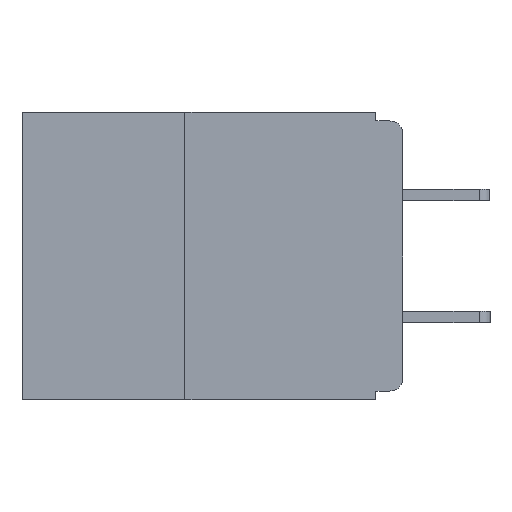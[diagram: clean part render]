
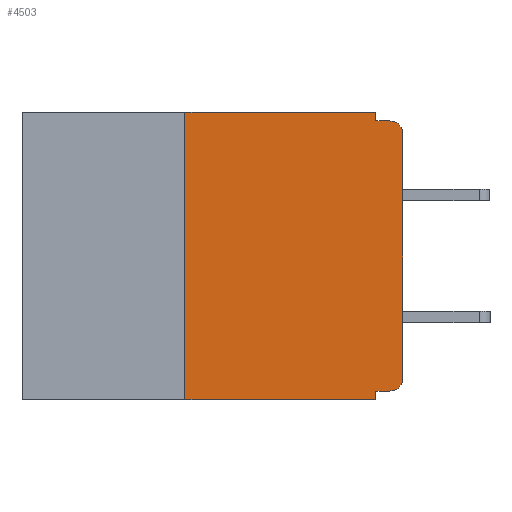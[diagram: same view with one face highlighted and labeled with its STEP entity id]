
A CAD part, left-side view. The second image highlights one B-rep face of the part: STEP entity #4503.
In plain terms, the highlighted planar face has unit normal (-1, 0, 0).
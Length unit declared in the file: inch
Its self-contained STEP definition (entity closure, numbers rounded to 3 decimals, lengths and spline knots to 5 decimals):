
#257 = VERTEX_POINT ( 'NONE', #8727 ) ;
#438 = FACE_OUTER_BOUND ( 'NONE', #10546, .T. ) ;
#1735 = CARTESIAN_POINT ( 'NONE',  ( 0., 0.437, 0. ) ) ;
#1757 = LINE ( 'NONE', #1735, #21112 ) ;
#1858 = LINE ( 'NONE', #15190, #22020 ) ;
#2003 = DIRECTION ( 'NONE',  ( 0., -1., 0. ) ) ;
#3156 = CARTESIAN_POINT ( 'NONE',  ( 0., 0.25, 0. ) ) ;
#3162 = VECTOR ( 'NONE', #19032, 39.37008 ) ;
#3169 = DIRECTION ( 'NONE',  ( 0., 0., -1. ) ) ;
#3252 = ORIENTED_EDGE ( 'NONE', *, *, #29074, .T. ) ;
#3434 = CIRCLE ( 'NONE', #23479, 0.015 ) ;
#4366 = EDGE_CURVE ( 'NONE', #22502, #10629, #18599, .T. ) ;
#4446 = AXIS2_PLACEMENT_3D ( 'NONE', #15179, #31533, #14517 ) ;
#4468 = CARTESIAN_POINT ( 'NONE',  ( 0., 0.031, -0.32 ) ) ;
#4503 = ADVANCED_FACE ( 'NONE', ( #438 ), #16304, .F. ) ;
#4545 = VECTOR ( 'NONE', #31366, 39.37008 ) ;
#5635 = CARTESIAN_POINT ( 'NONE',  ( 0., 0.015, -0.025 ) ) ;
#5752 = CARTESIAN_POINT ( 'NONE',  ( 0., 0.031, 0. ) ) ;
#6085 = VECTOR ( 'NONE', #2003, 39.37008 ) ;
#6101 = VERTEX_POINT ( 'NONE', #30113 ) ;
#7073 = DIRECTION ( 'NONE',  ( 0., -1., 0. ) ) ;
#8276 = ORIENTED_EDGE ( 'NONE', *, *, #32309, .T. ) ;
#8332 = DIRECTION ( 'NONE',  ( 0., 0., -1. ) ) ;
#8727 = CARTESIAN_POINT ( 'NONE',  ( 0., 0.015, -0.01 ) ) ;
#9222 = CARTESIAN_POINT ( 'NONE',  ( 0., 0., -0.025 ) ) ;
#9462 = ORIENTED_EDGE ( 'NONE', *, *, #4366, .F. ) ;
#10222 = LINE ( 'NONE', #30725, #30030 ) ;
#10264 = ORIENTED_EDGE ( 'NONE', *, *, #11863, .T. ) ;
#10299 = EDGE_CURVE ( 'NONE', #20189, #31922, #17221, .T. ) ;
#10546 = EDGE_LOOP ( 'NONE', ( #3252, #17311, #31703, #18929, #33230, #13656, #8276, #28941, #9462, #10264 ) ) ;
#10629 = VERTEX_POINT ( 'NONE', #4468 ) ;
#11338 = CIRCLE ( 'NONE', #29171, 0.015 ) ;
#11863 = EDGE_CURVE ( 'NONE', #22502, #19677, #11338, .T. ) ;
#12012 = CARTESIAN_POINT ( 'NONE',  ( 0., 0.031, 0. ) ) ;
#12367 = VECTOR ( 'NONE', #30025, 39.37008 ) ;
#13142 = LINE ( 'NONE', #17785, #6085 ) ;
#13295 = CARTESIAN_POINT ( 'NONE',  ( 0., 0.031, -0.33 ) ) ;
#13656 = ORIENTED_EDGE ( 'NONE', *, *, #10299, .F. ) ;
#13784 = EDGE_CURVE ( 'NONE', #6101, #257, #1858, .T. ) ;
#14517 = DIRECTION ( 'NONE',  ( 0., 0., -1. ) ) ;
#14643 = EDGE_CURVE ( 'NONE', #16008, #257, #3434, .T. ) ;
#15179 = CARTESIAN_POINT ( 'NONE',  ( 0., 0.437, 0. ) ) ;
#15190 = CARTESIAN_POINT ( 'NONE',  ( 0., 0., -0.01 ) ) ;
#15441 = DIRECTION ( 'NONE',  ( -1., 0., 0. ) ) ;
#15709 = VERTEX_POINT ( 'NONE', #13295 ) ;
#15822 = EDGE_CURVE ( 'NONE', #10629, #15709, #29813, .T. ) ;
#16008 = VERTEX_POINT ( 'NONE', #9222 ) ;
#16304 = PLANE ( 'NONE',  #4446 ) ;
#16428 = CARTESIAN_POINT ( 'NONE',  ( 0., 0.25, -0.33 ) ) ;
#17011 = VECTOR ( 'NONE', #3169, 39.37008 ) ;
#17221 = LINE ( 'NONE', #16428, #3162 ) ;
#17311 = ORIENTED_EDGE ( 'NONE', *, *, #14643, .T. ) ;
#17783 = DIRECTION ( 'NONE',  ( 0., -1., 0. ) ) ;
#17785 = CARTESIAN_POINT ( 'NONE',  ( 0., 0.437, -0.33 ) ) ;
#18599 = LINE ( 'NONE', #28818, #4545 ) ;
#18929 = ORIENTED_EDGE ( 'NONE', *, *, #31501, .F. ) ;
#18960 = CARTESIAN_POINT ( 'NONE',  ( 0., 0.031, -0.33 ) ) ;
#19032 = DIRECTION ( 'NONE',  ( 0., 0., 1. ) ) ;
#19357 = CARTESIAN_POINT ( 'NONE',  ( 0., 0.25, -0.33 ) ) ;
#19677 = VERTEX_POINT ( 'NONE', #29996 ) ;
#20189 = VERTEX_POINT ( 'NONE', #19357 ) ;
#20831 = CARTESIAN_POINT ( 'NONE',  ( 0., 0.015, -0.32 ) ) ;
#21112 = VECTOR ( 'NONE', #7073, 39.37008 ) ;
#22020 = VECTOR ( 'NONE', #17783, 39.37008 ) ;
#22502 = VERTEX_POINT ( 'NONE', #20831 ) ;
#23162 = DIRECTION ( 'NONE',  ( 0., 0., 1. ) ) ;
#23479 = AXIS2_PLACEMENT_3D ( 'NONE', #5635, #23941, #8332 ) ;
#23941 = DIRECTION ( 'NONE',  ( -1., 0., 0. ) ) ;
#25441 = EDGE_CURVE ( 'NONE', #31922, #25766, #1757, .T. ) ;
#25766 = VERTEX_POINT ( 'NONE', #5752 ) ;
#28818 = CARTESIAN_POINT ( 'NONE',  ( 0., 0., -0.32 ) ) ;
#28941 = ORIENTED_EDGE ( 'NONE', *, *, #15822, .F. ) ;
#29074 = EDGE_CURVE ( 'NONE', #19677, #16008, #10222, .T. ) ;
#29171 = AXIS2_PLACEMENT_3D ( 'NONE', #30780, #15441, #33263 ) ;
#29813 = LINE ( 'NONE', #18960, #17011 ) ;
#29996 = CARTESIAN_POINT ( 'NONE',  ( 0., 0., -0.305 ) ) ;
#30025 = DIRECTION ( 'NONE',  ( 0., 0., -1. ) ) ;
#30030 = VECTOR ( 'NONE', #23162, 39.37008 ) ;
#30113 = CARTESIAN_POINT ( 'NONE',  ( 0., 0.031, -0.01 ) ) ;
#30725 = CARTESIAN_POINT ( 'NONE',  ( 0., 0., 0. ) ) ;
#30780 = CARTESIAN_POINT ( 'NONE',  ( 0., 0.015, -0.305 ) ) ;
#31366 = DIRECTION ( 'NONE',  ( 0., 1., 0. ) ) ;
#31501 = EDGE_CURVE ( 'NONE', #25766, #6101, #32055, .T. ) ;
#31533 = DIRECTION ( 'NONE',  ( 1., 0., 0. ) ) ;
#31703 = ORIENTED_EDGE ( 'NONE', *, *, #13784, .F. ) ;
#31922 = VERTEX_POINT ( 'NONE', #3156 ) ;
#32055 = LINE ( 'NONE', #12012, #12367 ) ;
#32309 = EDGE_CURVE ( 'NONE', #20189, #15709, #13142, .T. ) ;
#33230 = ORIENTED_EDGE ( 'NONE', *, *, #25441, .F. ) ;
#33263 = DIRECTION ( 'NONE',  ( 0., 0., -1. ) ) ;
